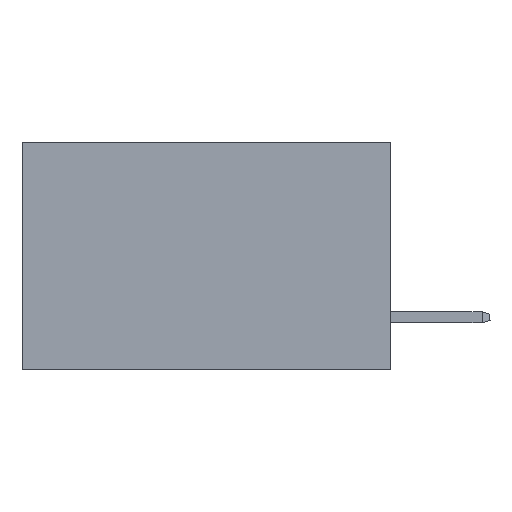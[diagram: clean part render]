
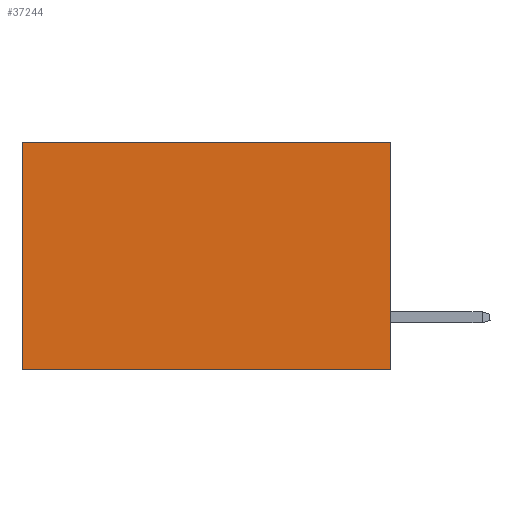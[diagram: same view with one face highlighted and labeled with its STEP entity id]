
A CAD part, left-side view. The second image highlights one B-rep face of the part: STEP entity #37244.
In plain terms, the highlighted planar face has unit normal (-1, 0, 0).
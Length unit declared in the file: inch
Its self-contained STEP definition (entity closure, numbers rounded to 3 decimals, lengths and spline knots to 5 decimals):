
#2845 = VERTEX_POINT ( 'NONE', #22032 ) ;
#3788 = ORIENTED_EDGE ( 'NONE', *, *, #18075, .F. ) ;
#3792 = CARTESIAN_POINT ( 'NONE',  ( 0.2875, 0., 0. ) ) ;
#4307 = CARTESIAN_POINT ( 'NONE',  ( 0.2875, 0.6, 0. ) ) ;
#4366 = DIRECTION ( 'NONE',  ( 1., 0., 0. ) ) ;
#4610 = ORIENTED_EDGE ( 'NONE', *, *, #11219, .T. ) ;
#6547 = EDGE_CURVE ( 'NONE', #2845, #28877, #8041, .T. ) ;
#6983 = CARTESIAN_POINT ( 'NONE',  ( 0.2875, 0.6, -0.37 ) ) ;
#7974 = DIRECTION ( 'NONE',  ( 0., 0., -1. ) ) ;
#8041 = LINE ( 'NONE', #11847, #29380 ) ;
#8611 = FACE_OUTER_BOUND ( 'NONE', #23220, .T. ) ;
#10576 = VERTEX_POINT ( 'NONE', #4307 ) ;
#10720 = VECTOR ( 'NONE', #13889, 39.37008 ) ;
#11200 = LINE ( 'NONE', #25592, #10720 ) ;
#11219 = EDGE_CURVE ( 'NONE', #10576, #28877, #11200, .T. ) ;
#11847 = CARTESIAN_POINT ( 'NONE',  ( 0.2875, 0., -0.37 ) ) ;
#13377 = DIRECTION ( 'NONE',  ( 0., 0., -1. ) ) ;
#13889 = DIRECTION ( 'NONE',  ( 0., 0., -1. ) ) ;
#14967 = LINE ( 'NONE', #33267, #36896 ) ;
#16193 = VERTEX_POINT ( 'NONE', #37429 ) ;
#17970 = VECTOR ( 'NONE', #34951, 39.37008 ) ;
#18075 = EDGE_CURVE ( 'NONE', #16193, #2845, #14967, .T. ) ;
#18393 = DIRECTION ( 'NONE',  ( 0., 1., 0. ) ) ;
#18956 = LINE ( 'NONE', #40727, #17970 ) ;
#22032 = CARTESIAN_POINT ( 'NONE',  ( 0.2875, 0., -0.37 ) ) ;
#23220 = EDGE_LOOP ( 'NONE', ( #4610, #37829, #3788, #29910 ) ) ;
#25592 = CARTESIAN_POINT ( 'NONE',  ( 0.2875, 0.6, 0. ) ) ;
#28877 = VERTEX_POINT ( 'NONE', #6983 ) ;
#29380 = VECTOR ( 'NONE', #18393, 39.37008 ) ;
#29910 = ORIENTED_EDGE ( 'NONE', *, *, #38150, .T. ) ;
#32524 = AXIS2_PLACEMENT_3D ( 'NONE', #3792, #4366, #13377 ) ;
#32839 = PLANE ( 'NONE',  #32524 ) ;
#33267 = CARTESIAN_POINT ( 'NONE',  ( 0.2875, 0., 0. ) ) ;
#34951 = DIRECTION ( 'NONE',  ( 0., 1., 0. ) ) ;
#36896 = VECTOR ( 'NONE', #7974, 39.37008 ) ;
#37244 = ADVANCED_FACE ( 'NONE', ( #8611 ), #32839, .F. ) ;
#37429 = CARTESIAN_POINT ( 'NONE',  ( 0.2875, 0., 0. ) ) ;
#37829 = ORIENTED_EDGE ( 'NONE', *, *, #6547, .F. ) ;
#38150 = EDGE_CURVE ( 'NONE', #16193, #10576, #18956, .T. ) ;
#40727 = CARTESIAN_POINT ( 'NONE',  ( 0.2875, 0., 0. ) ) ;
